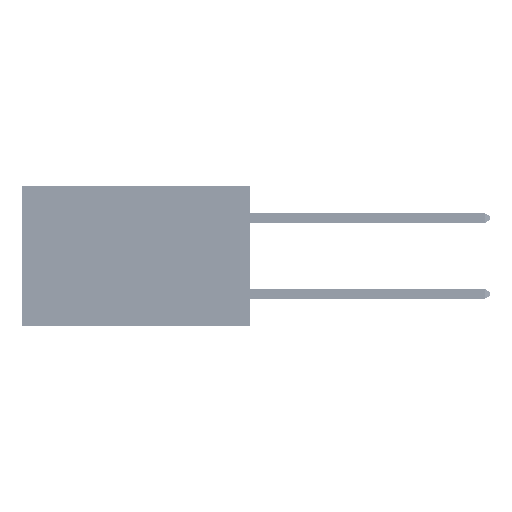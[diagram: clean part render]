
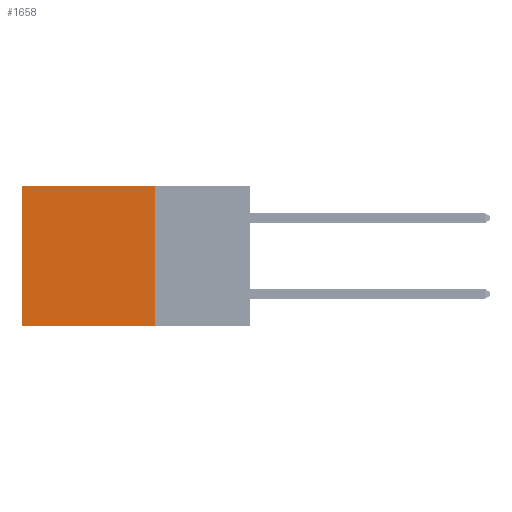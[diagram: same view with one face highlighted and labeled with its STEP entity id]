
A CAD part, left-side view. The second image highlights one B-rep face of the part: STEP entity #1658.
In plain terms, the highlighted planar face has unit normal (-1, 0, 0).
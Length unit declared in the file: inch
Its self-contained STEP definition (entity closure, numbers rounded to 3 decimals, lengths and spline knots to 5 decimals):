
#1469 = ORIENTED_EDGE ( 'NONE', *, *, #10639, .T. ) ;
#1658 = ADVANCED_FACE ( 'NONE', ( #13716 ), #2084, .F. ) ;
#2084 = PLANE ( 'NONE',  #47620 ) ;
#2250 = DIRECTION ( 'NONE',  ( 0., 0., -1. ) ) ;
#3968 = CARTESIAN_POINT ( 'NONE',  ( 0.2875, 0.6, 0. ) ) ;
#5580 = CARTESIAN_POINT ( 'NONE',  ( 0.2875, 0.25, 0. ) ) ;
#5777 = DIRECTION ( 'NONE',  ( 0., 1., 0. ) ) ;
#10350 = ORIENTED_EDGE ( 'NONE', *, *, #42926, .F. ) ;
#10409 = CARTESIAN_POINT ( 'NONE',  ( 0.2875, 0.25, 0. ) ) ;
#10639 = EDGE_CURVE ( 'NONE', #16036, #34880, #30721, .T. ) ;
#11071 = EDGE_CURVE ( 'NONE', #16036, #45867, #20271, .T. ) ;
#13418 = VERTEX_POINT ( 'NONE', #21987 ) ;
#13716 = FACE_OUTER_BOUND ( 'NONE', #33399, .T. ) ;
#14101 = CARTESIAN_POINT ( 'NONE',  ( 0.2875, 0.25, -0.37 ) ) ;
#15984 = EDGE_CURVE ( 'NONE', #34880, #13418, #31380, .T. ) ;
#16036 = VERTEX_POINT ( 'NONE', #44252 ) ;
#16419 = DIRECTION ( 'NONE',  ( 0., 0., -1. ) ) ;
#20271 = LINE ( 'NONE', #28070, #47716 ) ;
#21010 = VECTOR ( 'NONE', #32667, 39.37008 ) ;
#21987 = CARTESIAN_POINT ( 'NONE',  ( 0.2875, 0.6, -0.37 ) ) ;
#24642 = CARTESIAN_POINT ( 'NONE',  ( 0.2875, 0.6, 0. ) ) ;
#25310 = CARTESIAN_POINT ( 'NONE',  ( 0.2875, 0.25, -0.37 ) ) ;
#25650 = DIRECTION ( 'NONE',  ( 1., 0., 0. ) ) ;
#28070 = CARTESIAN_POINT ( 'NONE',  ( 0.2875, 0.25, 0. ) ) ;
#30721 = LINE ( 'NONE', #5580, #44101 ) ;
#31380 = LINE ( 'NONE', #24642, #21010 ) ;
#32667 = DIRECTION ( 'NONE',  ( 0., 0., -1. ) ) ;
#33057 = DIRECTION ( 'NONE',  ( 0., 1., 0. ) ) ;
#33399 = EDGE_LOOP ( 'NONE', ( #33573, #10350, #46945, #1469 ) ) ;
#33573 = ORIENTED_EDGE ( 'NONE', *, *, #15984, .T. ) ;
#34880 = VERTEX_POINT ( 'NONE', #3968 ) ;
#36404 = VECTOR ( 'NONE', #5777, 39.37008 ) ;
#40061 = LINE ( 'NONE', #14101, #36404 ) ;
#42926 = EDGE_CURVE ( 'NONE', #45867, #13418, #40061, .T. ) ;
#44101 = VECTOR ( 'NONE', #33057, 39.37008 ) ;
#44252 = CARTESIAN_POINT ( 'NONE',  ( 0.2875, 0.25, 0. ) ) ;
#45867 = VERTEX_POINT ( 'NONE', #25310 ) ;
#46945 = ORIENTED_EDGE ( 'NONE', *, *, #11071, .F. ) ;
#47620 = AXIS2_PLACEMENT_3D ( 'NONE', #10409, #25650, #2250 ) ;
#47716 = VECTOR ( 'NONE', #16419, 39.37008 ) ;
